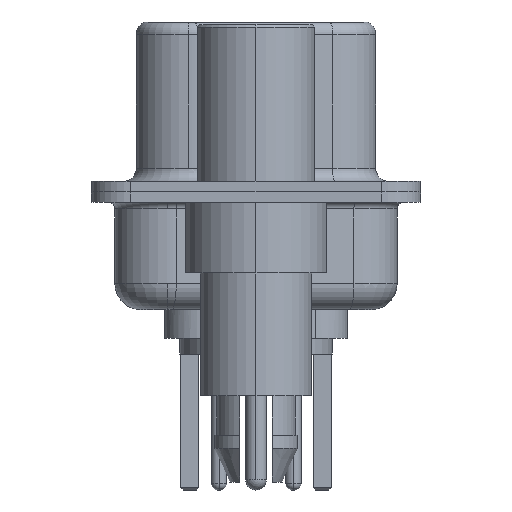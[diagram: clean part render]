
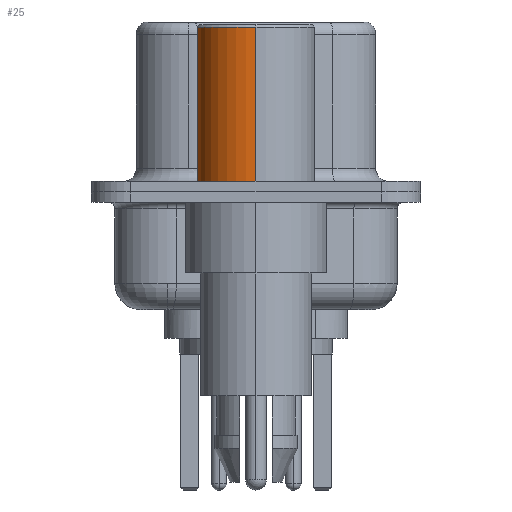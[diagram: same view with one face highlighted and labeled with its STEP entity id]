
A CAD part, left-side view. The second image highlights one B-rep face of the part: STEP entity #25.
In plain terms, the highlighted cylindrical face has radius 2.25 mm (diameter 4.5 mm), a partial arc.
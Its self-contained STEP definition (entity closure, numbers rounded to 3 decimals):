
#25 = ADVANCED_FACE ( 'NONE', ( #5621 ), #5155, .T. ) ;
#68 = LINE ( 'NONE', #17787, #3220 ) ;
#729 = DIRECTION ( 'NONE',  ( 0., 0., 1. ) ) ;
#1759 = LINE ( 'NONE', #7673, #5885 ) ;
#2108 = EDGE_LOOP ( 'NONE', ( #15800, #6738, #10988, #6276 ) ) ;
#2470 = CIRCLE ( 'NONE', #6223, 2.25 ) ;
#3201 = DIRECTION ( 'NONE',  ( 0., 0., 1. ) ) ;
#3220 = VECTOR ( 'NONE', #729, 1000. ) ;
#3928 = EDGE_CURVE ( 'NONE', #19338, #8475, #15691, .T. ) ;
#5155 = CYLINDRICAL_SURFACE ( 'NONE', #15962, 2.25 ) ;
#5621 = FACE_OUTER_BOUND ( 'NONE', #2108, .T. ) ;
#5885 = VECTOR ( 'NONE', #16985, 1000. ) ;
#6223 = AXIS2_PLACEMENT_3D ( 'NONE', #12525, #3201, #14105 ) ;
#6276 = ORIENTED_EDGE ( 'NONE', *, *, #15802, .F. ) ;
#6400 = CARTESIAN_POINT ( 'NONE',  ( 2.25, 0., 6.3 ) ) ;
#6445 = VERTEX_POINT ( 'NONE', #12440 ) ;
#6738 = ORIENTED_EDGE ( 'NONE', *, *, #16160, .T. ) ;
#7336 = DIRECTION ( 'NONE',  ( 0., 0., 1. ) ) ;
#7673 = CARTESIAN_POINT ( 'NONE',  ( 2.25, 0., 0.581 ) ) ;
#8104 = CARTESIAN_POINT ( 'NONE',  ( 0., 0., 6.3 ) ) ;
#8475 = VERTEX_POINT ( 'NONE', #18422 ) ;
#10640 = EDGE_CURVE ( 'NONE', #11078, #6445, #2470, .T. ) ;
#10838 = AXIS2_PLACEMENT_3D ( 'NONE', #8104, #7336, #17299 ) ;
#10988 = ORIENTED_EDGE ( 'NONE', *, *, #3928, .F. ) ;
#11078 = VERTEX_POINT ( 'NONE', #12231 ) ;
#12231 = CARTESIAN_POINT ( 'NONE',  ( 2.25, 0., 0.4 ) ) ;
#12440 = CARTESIAN_POINT ( 'NONE',  ( -2.25, 0., 0.4 ) ) ;
#12525 = CARTESIAN_POINT ( 'NONE',  ( 0., 0., 0.4 ) ) ;
#14103 = DIRECTION ( 'NONE',  ( 0., 0., 1. ) ) ;
#14105 = DIRECTION ( 'NONE',  ( 1., 0., 0. ) ) ;
#14138 = CARTESIAN_POINT ( 'NONE',  ( 0., 0., 0.581 ) ) ;
#15691 = CIRCLE ( 'NONE', #10838, 2.25 ) ;
#15800 = ORIENTED_EDGE ( 'NONE', *, *, #10640, .T. ) ;
#15802 = EDGE_CURVE ( 'NONE', #11078, #19338, #1759, .T. ) ;
#15962 = AXIS2_PLACEMENT_3D ( 'NONE', #14138, #14103, #17616 ) ;
#16160 = EDGE_CURVE ( 'NONE', #6445, #8475, #68, .T. ) ;
#16985 = DIRECTION ( 'NONE',  ( 0., 0., 1. ) ) ;
#17299 = DIRECTION ( 'NONE',  ( 1., 0., 0. ) ) ;
#17616 = DIRECTION ( 'NONE',  ( 1., 0., 0. ) ) ;
#17787 = CARTESIAN_POINT ( 'NONE',  ( -2.25, 0., 0.581 ) ) ;
#18422 = CARTESIAN_POINT ( 'NONE',  ( -2.25, 0., 6.3 ) ) ;
#19338 = VERTEX_POINT ( 'NONE', #6400 ) ;
